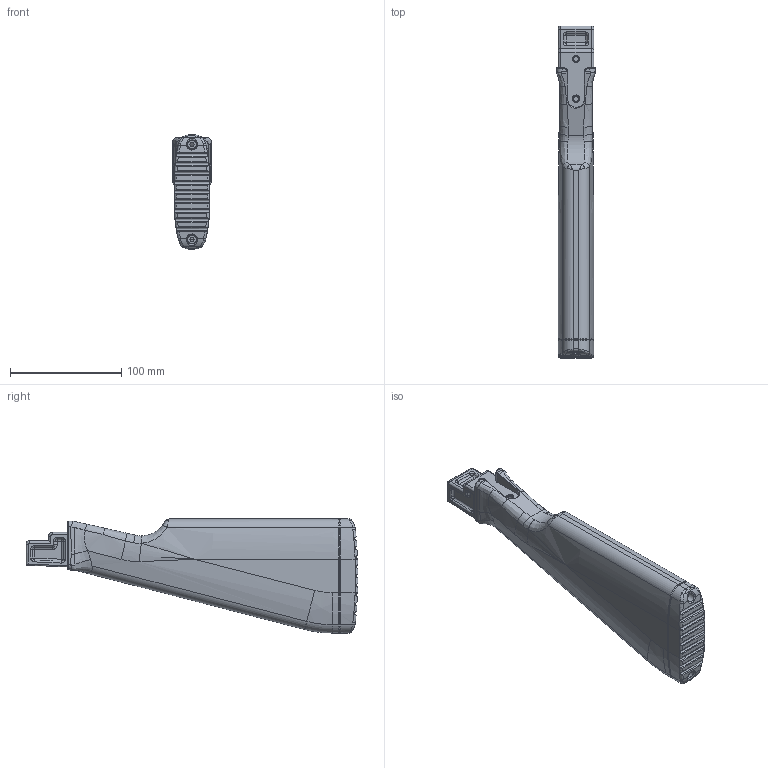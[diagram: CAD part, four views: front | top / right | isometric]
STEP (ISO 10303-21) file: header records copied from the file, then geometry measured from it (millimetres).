
FILE_DESCRIPTION(/* description */ (''),/* implementation_level */ '2;1');
FILE_NAME(/* name */ 'Single Piece Stock.step',/* time_stamp */ '2021-09-27T04:30:23-04:00',/* author */ (''),/* organization */ (''),/* preprocessor_version */ 'ST-DEVELOPER v18.1',/* originating_system */ 'Autodesk Translation Framework v10.10.0.1391',/* authorisation */ '');
FILE_SCHEMA (('AUTOMOTIVE_DESIGN { 1 0 10303 214 3 1 1 }'));
Length unit declared in the file: millimetre
Products named in the file (1): Single Piece Stock
Bounding box: 35 x 298.17 x 102.57 mm (x, y, z)
Volume: 324342.6 mm3; surface area: 97339.7 mm2
Topology: 2 solids, 2 shells, 659 faces, 1569 edges, 906 vertices
Faces by surface type: bspline 231, cylinder 207, plane 79, torus 76, cone 42, sphere 24
Full cylindrical faces by diameter (mm): 3.7 x4, 4.6 x2, 8 x2
Entity records: 49227 total; most frequent: CARTESIAN_POINT 35359, ORIENTED_EDGE 3106, DIRECTION 2544, EDGE_CURVE 1553, AXIS2_PLACEMENT_3D 1046, VERTEX_POINT 906, EDGE_LOOP 677, FACE_OUTER_BOUND 659
